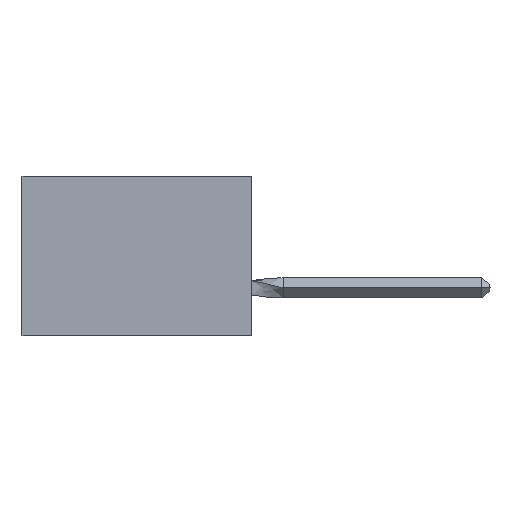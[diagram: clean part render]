
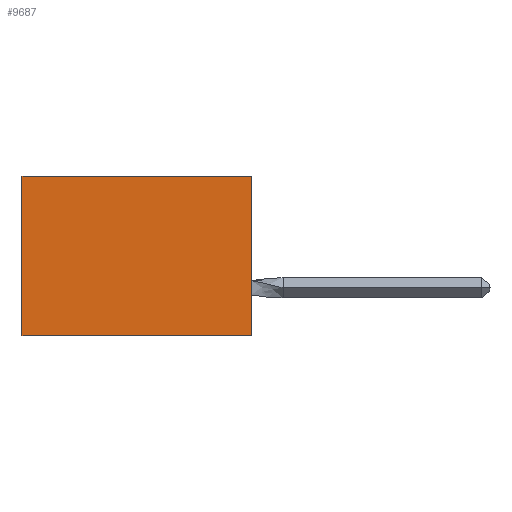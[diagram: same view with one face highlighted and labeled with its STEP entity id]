
A CAD part, left-side view. The second image highlights one B-rep face of the part: STEP entity #9687.
In plain terms, the highlighted planar face has unit normal (-1, 0, 0).
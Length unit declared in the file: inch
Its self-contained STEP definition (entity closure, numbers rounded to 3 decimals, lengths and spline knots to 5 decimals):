
#22 = VERTEX_POINT ( 'NONE', #17326 ) ;
#336 = DIRECTION ( 'NONE',  ( 0., 1., 0. ) ) ;
#1146 = CARTESIAN_POINT ( 'NONE',  ( 0.305, 0., -0.5 ) ) ;
#1216 = EDGE_CURVE ( 'NONE', #19233, #22, #7682, .T. ) ;
#1262 = ORIENTED_EDGE ( 'NONE', *, *, #10192, .T. ) ;
#2568 = DIRECTION ( 'NONE',  ( 0., 0., -1. ) ) ;
#2613 = CARTESIAN_POINT ( 'NONE',  ( 0.305, 0.72, 0. ) ) ;
#3370 = CARTESIAN_POINT ( 'NONE',  ( 0.305, 0., -0.5 ) ) ;
#4241 = CARTESIAN_POINT ( 'NONE',  ( 0.305, 0.72, -0.5 ) ) ;
#6265 = DIRECTION ( 'NONE',  ( 1., 0., 0. ) ) ;
#6434 = AXIS2_PLACEMENT_3D ( 'NONE', #16502, #6265, #2568 ) ;
#7307 = ORIENTED_EDGE ( 'NONE', *, *, #1216, .F. ) ;
#7682 = LINE ( 'NONE', #14032, #11106 ) ;
#8022 = ORIENTED_EDGE ( 'NONE', *, *, #22029, .T. ) ;
#8246 = CARTESIAN_POINT ( 'NONE',  ( 0.305, 0., 0. ) ) ;
#9047 = CARTESIAN_POINT ( 'NONE',  ( 0.305, 0., 0. ) ) ;
#9481 = DIRECTION ( 'NONE',  ( 0., 0., -1. ) ) ;
#9687 = ADVANCED_FACE ( 'NONE', ( #20895 ), #18100, .F. ) ;
#9692 = DIRECTION ( 'NONE',  ( 0., 0., -1. ) ) ;
#10192 = EDGE_CURVE ( 'NONE', #13331, #22, #15205, .T. ) ;
#10547 = DIRECTION ( 'NONE',  ( 0., 1., 0. ) ) ;
#11106 = VECTOR ( 'NONE', #336, 39.37008 ) ;
#13231 = ORIENTED_EDGE ( 'NONE', *, *, #14746, .F. ) ;
#13331 = VERTEX_POINT ( 'NONE', #2613 ) ;
#13493 = VECTOR ( 'NONE', #9692, 39.37008 ) ;
#13764 = LINE ( 'NONE', #1146, #13493 ) ;
#14032 = CARTESIAN_POINT ( 'NONE',  ( 0.305, 0., -0.5 ) ) ;
#14458 = EDGE_LOOP ( 'NONE', ( #1262, #7307, #13231, #8022 ) ) ;
#14746 = EDGE_CURVE ( 'NONE', #18179, #19233, #13764, .T. ) ;
#15205 = LINE ( 'NONE', #4241, #21953 ) ;
#15453 = VECTOR ( 'NONE', #10547, 39.37008 ) ;
#16502 = CARTESIAN_POINT ( 'NONE',  ( 0.305, 0., -0.5 ) ) ;
#17326 = CARTESIAN_POINT ( 'NONE',  ( 0.305, 0.72, -0.5 ) ) ;
#18100 = PLANE ( 'NONE',  #6434 ) ;
#18179 = VERTEX_POINT ( 'NONE', #8246 ) ;
#19233 = VERTEX_POINT ( 'NONE', #3370 ) ;
#20025 = LINE ( 'NONE', #9047, #15453 ) ;
#20895 = FACE_OUTER_BOUND ( 'NONE', #14458, .T. ) ;
#21953 = VECTOR ( 'NONE', #9481, 39.37008 ) ;
#22029 = EDGE_CURVE ( 'NONE', #18179, #13331, #20025, .T. ) ;
